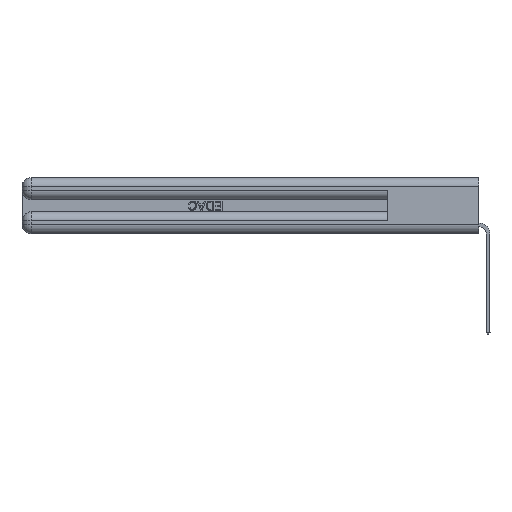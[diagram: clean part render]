
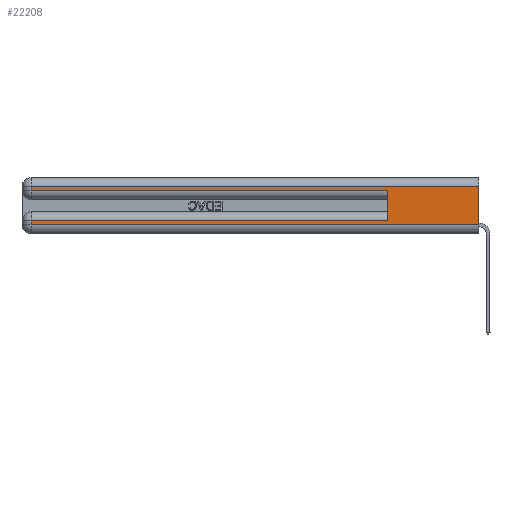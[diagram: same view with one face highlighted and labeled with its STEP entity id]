
A CAD part, left-side view. The second image highlights one B-rep face of the part: STEP entity #22208.
In plain terms, the highlighted planar face has unit normal (-1, 0, 0).
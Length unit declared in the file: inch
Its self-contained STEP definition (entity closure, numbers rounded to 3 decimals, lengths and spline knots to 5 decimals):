
#669 = CARTESIAN_POINT ( 'NONE',  ( 0., 2.94, 0.285 ) ) ;
#925 = EDGE_CURVE ( 'NONE', #24143, #10135, #3378, .T. ) ;
#1258 = FACE_OUTER_BOUND ( 'NONE', #14076, .T. ) ;
#1358 = DIRECTION ( 'NONE',  ( 0., 0., 1. ) ) ;
#1447 = ORIENTED_EDGE ( 'NONE', *, *, #2533, .T. ) ;
#1588 = EDGE_CURVE ( 'NONE', #17013, #10356, #25406, .T. ) ;
#2533 = EDGE_CURVE ( 'NONE', #10913, #3440, #15484, .T. ) ;
#2576 = CARTESIAN_POINT ( 'NONE',  ( 0., 2.94, 0.31 ) ) ;
#2651 = VECTOR ( 'NONE', #11907, 39.37008 ) ;
#3016 = VECTOR ( 'NONE', #16980, 39.37008 ) ;
#3113 = DIRECTION ( 'NONE',  ( 0., 0., -1. ) ) ;
#3280 = LINE ( 'NONE', #13857, #2651 ) ;
#3378 = LINE ( 'NONE', #23192, #20278 ) ;
#3440 = VERTEX_POINT ( 'NONE', #10547 ) ;
#4820 = DIRECTION ( 'NONE',  ( 0., 1., 0. ) ) ;
#5331 = DIRECTION ( 'NONE',  ( 0., 0., -1. ) ) ;
#6139 = CARTESIAN_POINT ( 'NONE',  ( 0., 2.94, 0.06 ) ) ;
#6438 = ORIENTED_EDGE ( 'NONE', *, *, #13547, .F. ) ;
#7755 = ORIENTED_EDGE ( 'NONE', *, *, #24196, .T. ) ;
#7847 = DIRECTION ( 'NONE',  ( 0., -1., 0. ) ) ;
#8155 = CARTESIAN_POINT ( 'NONE',  ( 0., 0., 0.37 ) ) ;
#8793 = CARTESIAN_POINT ( 'NONE',  ( 0., 0., 0.285 ) ) ;
#9869 = CARTESIAN_POINT ( 'NONE',  ( 0., 0.6, 0.085 ) ) ;
#10135 = VERTEX_POINT ( 'NONE', #2576 ) ;
#10356 = VERTEX_POINT ( 'NONE', #11469 ) ;
#10484 = ORIENTED_EDGE ( 'NONE', *, *, #11470, .T. ) ;
#10547 = CARTESIAN_POINT ( 'NONE',  ( 0., 0., 0.06 ) ) ;
#10754 = VECTOR ( 'NONE', #7847, 39.37008 ) ;
#10913 = VERTEX_POINT ( 'NONE', #6139 ) ;
#11102 = AXIS2_PLACEMENT_3D ( 'NONE', #8155, #24490, #12250 ) ;
#11469 = CARTESIAN_POINT ( 'NONE',  ( 0., 0.6, 0.285 ) ) ;
#11470 = EDGE_CURVE ( 'NONE', #10135, #17013, #3280, .T. ) ;
#11477 = VECTOR ( 'NONE', #5331, 39.37008 ) ;
#11907 = DIRECTION ( 'NONE',  ( 0., 0., -1. ) ) ;
#12048 = VECTOR ( 'NONE', #12437, 39.37008 ) ;
#12250 = DIRECTION ( 'NONE',  ( 0., 0., -1. ) ) ;
#12437 = DIRECTION ( 'NONE',  ( 0., 1., 0. ) ) ;
#12694 = LINE ( 'NONE', #24682, #12048 ) ;
#13547 = EDGE_CURVE ( 'NONE', #18541, #10356, #19427, .T. ) ;
#13585 = CARTESIAN_POINT ( 'NONE',  ( 0., 0.6, 0.145 ) ) ;
#13857 = CARTESIAN_POINT ( 'NONE',  ( 0., 2.94, 0.37 ) ) ;
#14076 = EDGE_LOOP ( 'NONE', ( #21929, #20950, #10484, #21452, #6438, #7755, #14518, #1447 ) ) ;
#14518 = ORIENTED_EDGE ( 'NONE', *, *, #18379, .T. ) ;
#14634 = VECTOR ( 'NONE', #1358, 39.37008 ) ;
#14952 = VERTEX_POINT ( 'NONE', #24595 ) ;
#15484 = LINE ( 'NONE', #26250, #10754 ) ;
#16171 = LINE ( 'NONE', #17380, #16840 ) ;
#16840 = VECTOR ( 'NONE', #3113, 39.37008 ) ;
#16901 = LINE ( 'NONE', #21564, #11477 ) ;
#16980 = DIRECTION ( 'NONE',  ( 0., -1., 0. ) ) ;
#17013 = VERTEX_POINT ( 'NONE', #669 ) ;
#17380 = CARTESIAN_POINT ( 'NONE',  ( 0., 0., 0.37 ) ) ;
#18379 = EDGE_CURVE ( 'NONE', #14952, #10913, #16901, .T. ) ;
#18541 = VERTEX_POINT ( 'NONE', #9869 ) ;
#19427 = LINE ( 'NONE', #13585, #14634 ) ;
#20278 = VECTOR ( 'NONE', #4820, 39.37008 ) ;
#20350 = PLANE ( 'NONE',  #11102 ) ;
#20950 = ORIENTED_EDGE ( 'NONE', *, *, #925, .T. ) ;
#21452 = ORIENTED_EDGE ( 'NONE', *, *, #1588, .T. ) ;
#21564 = CARTESIAN_POINT ( 'NONE',  ( 0., 2.94, 0.37 ) ) ;
#21929 = ORIENTED_EDGE ( 'NONE', *, *, #23132, .F. ) ;
#22208 = ADVANCED_FACE ( 'NONE', ( #1258 ), #20350, .F. ) ;
#23132 = EDGE_CURVE ( 'NONE', #24143, #3440, #16171, .T. ) ;
#23192 = CARTESIAN_POINT ( 'NONE',  ( 0., 0., 0.31 ) ) ;
#24143 = VERTEX_POINT ( 'NONE', #24495 ) ;
#24196 = EDGE_CURVE ( 'NONE', #18541, #14952, #12694, .T. ) ;
#24490 = DIRECTION ( 'NONE',  ( 1., 0., 0. ) ) ;
#24495 = CARTESIAN_POINT ( 'NONE',  ( 0., 0., 0.31 ) ) ;
#24595 = CARTESIAN_POINT ( 'NONE',  ( 0., 2.94, 0.085 ) ) ;
#24682 = CARTESIAN_POINT ( 'NONE',  ( 0., 0., 0.085 ) ) ;
#25406 = LINE ( 'NONE', #8793, #3016 ) ;
#26250 = CARTESIAN_POINT ( 'NONE',  ( 0., 0., 0.06 ) ) ;
